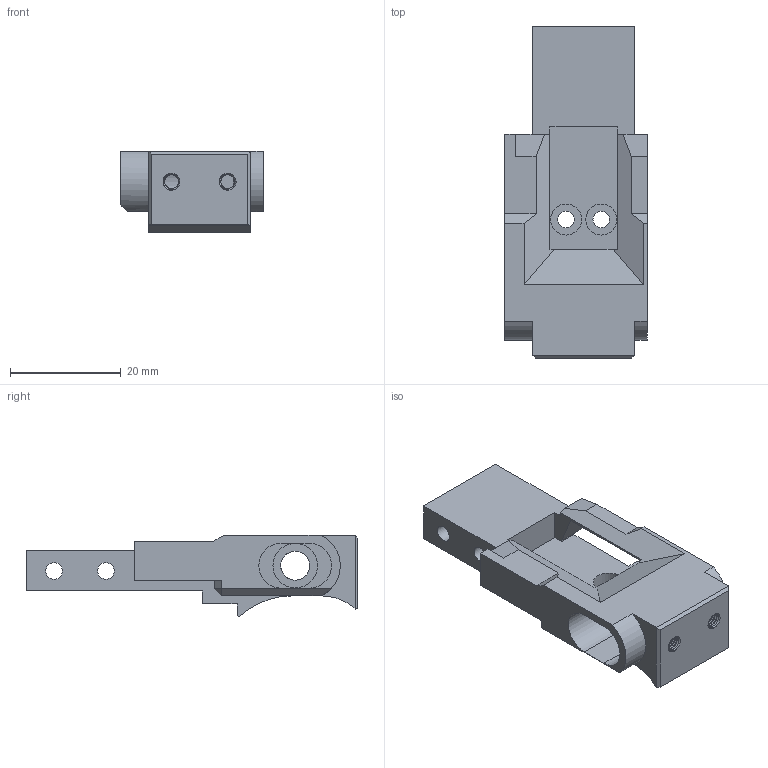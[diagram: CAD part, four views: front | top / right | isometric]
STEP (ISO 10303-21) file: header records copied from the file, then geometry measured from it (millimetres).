
FILE_DESCRIPTION(/* description */ (''),/* implementation_level */ '2;1');
FILE_NAME(/* name */ 'FCU Mag Catch Joiner 47.step',/* time_stamp */ '2024-01-16T15:57:47-05:00',/* author */ (''),/* organization */ (''),/* preprocessor_version */ 'ST-DEVELOPER v20',/* originating_system */ 'Autodesk Translation Framework v12.14.0.127',/* authorisation */ '');
FILE_SCHEMA (('AUTOMOTIVE_DESIGN { 1 0 10303 214 3 1 1 }'));
Length unit declared in the file: inch
Products named in the file (1): FCU Mag Catch Joiner 47
Bounding box: 25.79 x 59.98 x 14.66 mm (x, y, z)
Volume: 7801.9 mm3; surface area: 6212.1 mm2
Topology: 1 solids, 1 shells, 157 faces, 456 edges, 301 vertices
Faces by surface type: cylinder 77, plane 59, bspline 17, cone 4
Full cylindrical faces by diameter (mm): 2.529 x11, 3 x4, 3.086 x9, 5.258 x1, 5.6 x2, 8.052 x1
Entity records: 8303 total; most frequent: CARTESIAN_POINT 4453, ORIENTED_EDGE 912, DIRECTION 602, EDGE_CURVE 456, VERTEX_POINT 301, LINE 232, VECTOR 232, AXIS2_PLACEMENT_3D 185
